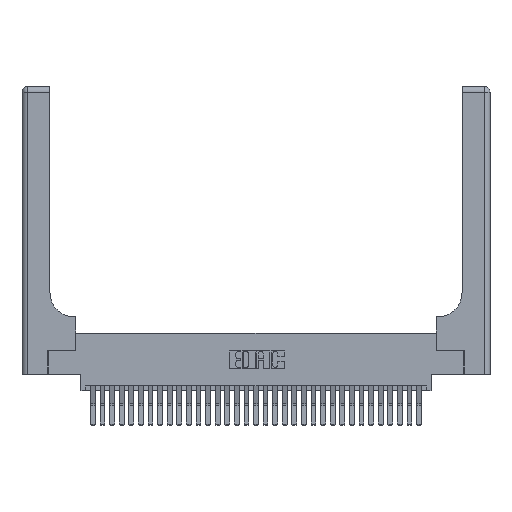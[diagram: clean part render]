
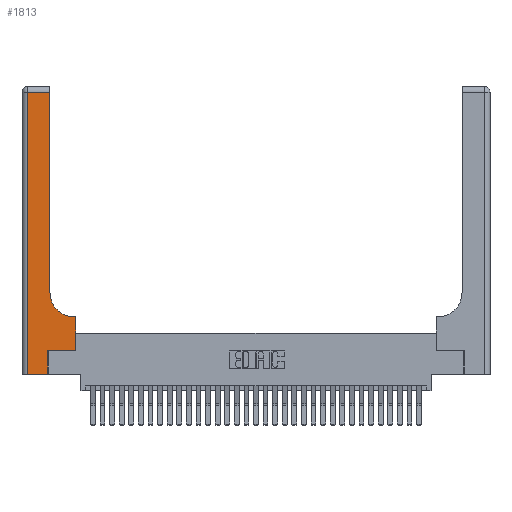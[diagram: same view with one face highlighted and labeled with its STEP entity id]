
A CAD part, top view. The second image highlights one B-rep face of the part: STEP entity #1813.
In plain terms, the highlighted planar face has unit normal (0, 0, 1).
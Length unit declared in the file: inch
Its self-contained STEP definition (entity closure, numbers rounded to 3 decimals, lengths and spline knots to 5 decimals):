
#61 = EDGE_LOOP ( 'NONE', ( #7370, #3159, #1020, #6423, #2488, #30501, #27086, #24970, #11320 ) ) ;
#1020 = ORIENTED_EDGE ( 'NONE', *, *, #25597, .T. ) ;
#1101 = VERTEX_POINT ( 'NONE', #14931 ) ;
#1113 = AXIS2_PLACEMENT_3D ( 'NONE', #30762, #17907, #20317 ) ;
#1400 = LINE ( 'NONE', #22677, #3424 ) ;
#1581 = CARTESIAN_POINT ( 'NONE',  ( 0., 0., 0.37 ) ) ;
#1813 = ADVANCED_FACE ( 'NONE', ( #24386 ), #12706, .F. ) ;
#2488 = ORIENTED_EDGE ( 'NONE', *, *, #22577, .T. ) ;
#3159 = ORIENTED_EDGE ( 'NONE', *, *, #16634, .T. ) ;
#3366 = EDGE_CURVE ( 'NONE', #14813, #20308, #11300, .T. ) ;
#3424 = VECTOR ( 'NONE', #16093, 39.37008 ) ;
#3567 = CARTESIAN_POINT ( 'NONE',  ( 0.269, 0.25, 0.37 ) ) ;
#3643 = DIRECTION ( 'NONE',  ( 1., 0., 0. ) ) ;
#4213 = VECTOR ( 'NONE', #16988, 39.37008 ) ;
#4403 = DIRECTION ( 'NONE',  ( -1., 0., 0. ) ) ;
#5188 = LINE ( 'NONE', #13958, #28079 ) ;
#6423 = ORIENTED_EDGE ( 'NONE', *, *, #29843, .T. ) ;
#6823 = CARTESIAN_POINT ( 'NONE',  ( 0.5585, 0.25, 0.37 ) ) ;
#7370 = ORIENTED_EDGE ( 'NONE', *, *, #12373, .T. ) ;
#7639 = CARTESIAN_POINT ( 'NONE',  ( 0.5585, 0.25, 0.37 ) ) ;
#7903 = EDGE_CURVE ( 'NONE', #32766, #9085, #26270, .T. ) ;
#8643 = DIRECTION ( 'NONE',  ( 1., 0., 0. ) ) ;
#9085 = VERTEX_POINT ( 'NONE', #19117 ) ;
#10143 = VERTEX_POINT ( 'NONE', #21255 ) ;
#10277 = CARTESIAN_POINT ( 'NONE',  ( 0., 2.94, 0.37 ) ) ;
#11230 = VERTEX_POINT ( 'NONE', #17469 ) ;
#11300 = CIRCLE ( 'NONE', #19491, 0.25 ) ;
#11320 = ORIENTED_EDGE ( 'NONE', *, *, #3366, .T. ) ;
#12373 = EDGE_CURVE ( 'NONE', #20308, #12984, #1400, .T. ) ;
#12706 = PLANE ( 'NONE',  #1113 ) ;
#12984 = VERTEX_POINT ( 'NONE', #32001 ) ;
#13644 = CARTESIAN_POINT ( 'NONE',  ( 0.269, 0., 0.37 ) ) ;
#13958 = CARTESIAN_POINT ( 'NONE',  ( 0.269, 0.25, 0.37 ) ) ;
#14813 = VERTEX_POINT ( 'NONE', #25663 ) ;
#14931 = CARTESIAN_POINT ( 'NONE',  ( 0.06, 0., 0.37 ) ) ;
#16093 = DIRECTION ( 'NONE',  ( 0., 1., 0. ) ) ;
#16366 = DIRECTION ( 'NONE',  ( 0., 1., 0. ) ) ;
#16374 = CARTESIAN_POINT ( 'NONE',  ( 0.5415, 0.85, 0.37 ) ) ;
#16634 = EDGE_CURVE ( 'NONE', #12984, #10143, #21557, .T. ) ;
#16988 = DIRECTION ( 'NONE',  ( 0., 1., 0. ) ) ;
#17065 = VERTEX_POINT ( 'NONE', #3567 ) ;
#17469 = CARTESIAN_POINT ( 'NONE',  ( 0.269, 0., 0.37 ) ) ;
#17629 = CARTESIAN_POINT ( 'NONE',  ( 0.06, 3., 0.37 ) ) ;
#17907 = DIRECTION ( 'NONE',  ( 0., 0., -1. ) ) ;
#18550 = VECTOR ( 'NONE', #28169, 39.37008 ) ;
#19117 = CARTESIAN_POINT ( 'NONE',  ( 0.5585, 0.6, 0.37 ) ) ;
#19491 = AXIS2_PLACEMENT_3D ( 'NONE', #16374, #21589, #8643 ) ;
#19936 = DIRECTION ( 'NONE',  ( 1., 0., 0. ) ) ;
#20308 = VERTEX_POINT ( 'NONE', #30645 ) ;
#20317 = DIRECTION ( 'NONE',  ( -1., 0., 0. ) ) ;
#20380 = CARTESIAN_POINT ( 'NONE',  ( 0.2915, 0.6, 0.37 ) ) ;
#21255 = CARTESIAN_POINT ( 'NONE',  ( 0.06, 2.94, 0.37 ) ) ;
#21557 = LINE ( 'NONE', #10277, #29378 ) ;
#21589 = DIRECTION ( 'NONE',  ( 0., 0., -1. ) ) ;
#21937 = LINE ( 'NONE', #1581, #32601 ) ;
#22577 = EDGE_CURVE ( 'NONE', #11230, #17065, #30291, .T. ) ;
#22677 = CARTESIAN_POINT ( 'NONE',  ( 0.2915, 3., 0.37 ) ) ;
#23787 = LINE ( 'NONE', #20380, #29967 ) ;
#24386 = FACE_OUTER_BOUND ( 'NONE', #61, .T. ) ;
#24591 = EDGE_CURVE ( 'NONE', #17065, #32766, #5188, .T. ) ;
#24970 = ORIENTED_EDGE ( 'NONE', *, *, #27344, .T. ) ;
#25597 = EDGE_CURVE ( 'NONE', #10143, #1101, #28413, .T. ) ;
#25663 = CARTESIAN_POINT ( 'NONE',  ( 0.5415, 0.6, 0.37 ) ) ;
#26270 = LINE ( 'NONE', #6823, #4213 ) ;
#27086 = ORIENTED_EDGE ( 'NONE', *, *, #7903, .T. ) ;
#27344 = EDGE_CURVE ( 'NONE', #9085, #14813, #23787, .T. ) ;
#28079 = VECTOR ( 'NONE', #3643, 39.37008 ) ;
#28169 = DIRECTION ( 'NONE',  ( 0., -1., 0. ) ) ;
#28413 = LINE ( 'NONE', #17629, #18550 ) ;
#29378 = VECTOR ( 'NONE', #33545, 39.37008 ) ;
#29843 = EDGE_CURVE ( 'NONE', #1101, #11230, #21937, .T. ) ;
#29967 = VECTOR ( 'NONE', #4403, 39.37008 ) ;
#30291 = LINE ( 'NONE', #13644, #31138 ) ;
#30501 = ORIENTED_EDGE ( 'NONE', *, *, #24591, .T. ) ;
#30645 = CARTESIAN_POINT ( 'NONE',  ( 0.2915, 0.85, 0.37 ) ) ;
#30762 = CARTESIAN_POINT ( 'NONE',  ( 0., 3., 0.37 ) ) ;
#31138 = VECTOR ( 'NONE', #16366, 39.37008 ) ;
#32001 = CARTESIAN_POINT ( 'NONE',  ( 0.2915, 2.94, 0.37 ) ) ;
#32601 = VECTOR ( 'NONE', #19936, 39.37008 ) ;
#32766 = VERTEX_POINT ( 'NONE', #7639 ) ;
#33545 = DIRECTION ( 'NONE',  ( -1., 0., 0. ) ) ;
